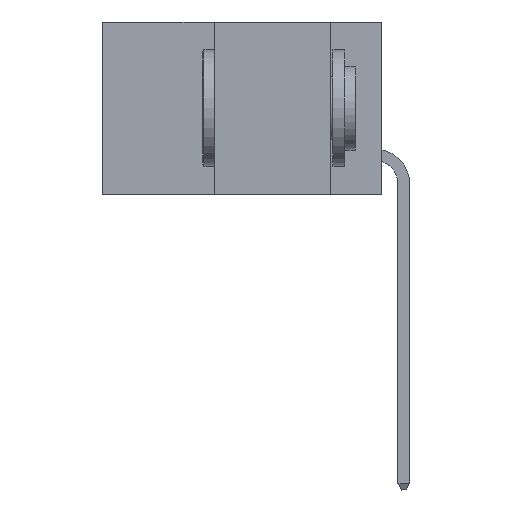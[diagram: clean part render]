
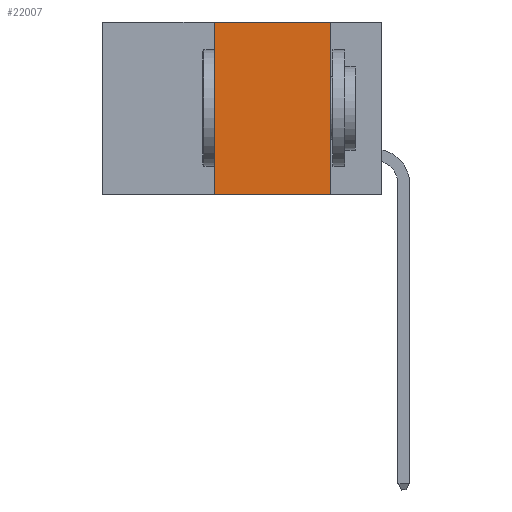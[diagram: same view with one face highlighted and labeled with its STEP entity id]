
A CAD part, left-side view. The second image highlights one B-rep face of the part: STEP entity #22007.
In plain terms, the highlighted planar face has unit normal (-1, 0, 0).
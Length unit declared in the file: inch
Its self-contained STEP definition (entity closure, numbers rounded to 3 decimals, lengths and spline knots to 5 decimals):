
#1182 = LINE ( 'NONE', #3570, #36483 ) ;
#3570 = CARTESIAN_POINT ( 'NONE',  ( 0., 0.6, 0. ) ) ;
#4376 = EDGE_CURVE ( 'NONE', #39160, #19004, #17077, .T. ) ;
#4849 = DIRECTION ( 'NONE',  ( 0., 0., -1. ) ) ;
#5302 = CARTESIAN_POINT ( 'NONE',  ( 0., 0.6, 0. ) ) ;
#5544 = CARTESIAN_POINT ( 'NONE',  ( 0., 0.11, 0. ) ) ;
#6572 = LINE ( 'NONE', #5544, #15045 ) ;
#7370 = ORIENTED_EDGE ( 'NONE', *, *, #25946, .F. ) ;
#7702 = VECTOR ( 'NONE', #13704, 39.37008 ) ;
#8813 = AXIS2_PLACEMENT_3D ( 'NONE', #5302, #18723, #4849 ) ;
#9312 = ORIENTED_EDGE ( 'NONE', *, *, #14188, .F. ) ;
#10934 = CARTESIAN_POINT ( 'NONE',  ( 0., 0.11, 0. ) ) ;
#12903 = EDGE_CURVE ( 'NONE', #39160, #28976, #20500, .T. ) ;
#13704 = DIRECTION ( 'NONE',  ( 0., -1., 0. ) ) ;
#14188 = EDGE_CURVE ( 'NONE', #22257, #28976, #6572, .T. ) ;
#15045 = VECTOR ( 'NONE', #39728, 39.37008 ) ;
#16027 = VECTOR ( 'NONE', #32414, 39.37008 ) ;
#17077 = LINE ( 'NONE', #18644, #16027 ) ;
#18644 = CARTESIAN_POINT ( 'NONE',  ( 0., 0.36, 0. ) ) ;
#18707 = CARTESIAN_POINT ( 'NONE',  ( 0., 0.11, -0.37 ) ) ;
#18723 = DIRECTION ( 'NONE',  ( 1., 0., 0. ) ) ;
#19004 = VERTEX_POINT ( 'NONE', #27160 ) ;
#19741 = CARTESIAN_POINT ( 'NONE',  ( 0., 0.36, -0.37 ) ) ;
#20500 = LINE ( 'NONE', #40877, #7702 ) ;
#20738 = DIRECTION ( 'NONE',  ( 0., -1., 0. ) ) ;
#22007 = ADVANCED_FACE ( 'NONE', ( #36230 ), #39017, .F. ) ;
#22257 = VERTEX_POINT ( 'NONE', #10934 ) ;
#24983 = EDGE_LOOP ( 'NONE', ( #9312, #7370, #44106, #39507 ) ) ;
#25946 = EDGE_CURVE ( 'NONE', #19004, #22257, #1182, .T. ) ;
#27160 = CARTESIAN_POINT ( 'NONE',  ( 0., 0.36, 0. ) ) ;
#28976 = VERTEX_POINT ( 'NONE', #18707 ) ;
#32414 = DIRECTION ( 'NONE',  ( 0., 0., 1. ) ) ;
#36230 = FACE_OUTER_BOUND ( 'NONE', #24983, .T. ) ;
#36483 = VECTOR ( 'NONE', #20738, 39.37008 ) ;
#39017 = PLANE ( 'NONE',  #8813 ) ;
#39160 = VERTEX_POINT ( 'NONE', #19741 ) ;
#39507 = ORIENTED_EDGE ( 'NONE', *, *, #12903, .T. ) ;
#39728 = DIRECTION ( 'NONE',  ( 0., 0., -1. ) ) ;
#40877 = CARTESIAN_POINT ( 'NONE',  ( 0., 0.6, -0.37 ) ) ;
#44106 = ORIENTED_EDGE ( 'NONE', *, *, #4376, .F. ) ;
